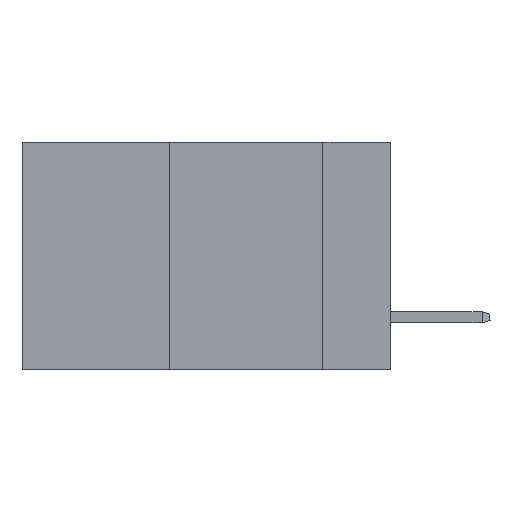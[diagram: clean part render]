
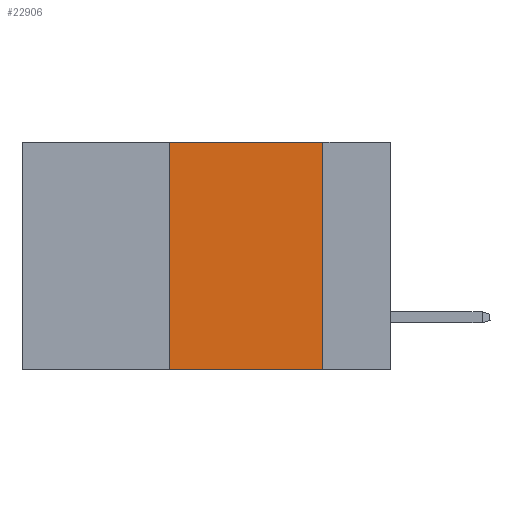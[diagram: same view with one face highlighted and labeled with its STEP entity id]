
A CAD part, left-side view. The second image highlights one B-rep face of the part: STEP entity #22906.
In plain terms, the highlighted planar face has unit normal (-1, 0, 0).
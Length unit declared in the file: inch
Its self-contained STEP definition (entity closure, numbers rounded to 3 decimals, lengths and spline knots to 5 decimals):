
#1070 = DIRECTION ( 'NONE',  ( 0., 0., 1. ) ) ;
#1856 = LINE ( 'NONE', #33654, #6864 ) ;
#2321 = CARTESIAN_POINT ( 'NONE',  ( 0., 0.6, -0.37 ) ) ;
#2967 = EDGE_CURVE ( 'NONE', #23604, #9490, #24756, .T. ) ;
#3745 = FACE_OUTER_BOUND ( 'NONE', #18576, .T. ) ;
#4186 = LINE ( 'NONE', #20845, #26300 ) ;
#4460 = DIRECTION ( 'NONE',  ( 1., 0., 0. ) ) ;
#4631 = EDGE_CURVE ( 'NONE', #9490, #32981, #4186, .T. ) ;
#6123 = EDGE_CURVE ( 'NONE', #23604, #20145, #26373, .T. ) ;
#6767 = DIRECTION ( 'NONE',  ( 0., 0., -1. ) ) ;
#6864 = VECTOR ( 'NONE', #6767, 39.37008 ) ;
#7736 = DIRECTION ( 'NONE',  ( 0., -1., 0. ) ) ;
#9490 = VERTEX_POINT ( 'NONE', #29292 ) ;
#10195 = VECTOR ( 'NONE', #7736, 39.37008 ) ;
#12508 = CARTESIAN_POINT ( 'NONE',  ( 0., 0.6, 0. ) ) ;
#13231 = ORIENTED_EDGE ( 'NONE', *, *, #25130, .F. ) ;
#15434 = ORIENTED_EDGE ( 'NONE', *, *, #4631, .F. ) ;
#16707 = CARTESIAN_POINT ( 'NONE',  ( 0., 0.11, 0. ) ) ;
#17453 = ORIENTED_EDGE ( 'NONE', *, *, #2967, .F. ) ;
#17587 = VECTOR ( 'NONE', #1070, 39.37008 ) ;
#18473 = CARTESIAN_POINT ( 'NONE',  ( 0., 0.11, -0.37 ) ) ;
#18576 = EDGE_LOOP ( 'NONE', ( #13231, #15434, #17453, #18637 ) ) ;
#18637 = ORIENTED_EDGE ( 'NONE', *, *, #6123, .T. ) ;
#20145 = VERTEX_POINT ( 'NONE', #18473 ) ;
#20845 = CARTESIAN_POINT ( 'NONE',  ( 0., 0.6, 0. ) ) ;
#22906 = ADVANCED_FACE ( 'NONE', ( #3745 ), #33245, .F. ) ;
#23501 = DIRECTION ( 'NONE',  ( 0., -1., 0. ) ) ;
#23604 = VERTEX_POINT ( 'NONE', #29286 ) ;
#24595 = CARTESIAN_POINT ( 'NONE',  ( 0., 0.36, 0. ) ) ;
#24756 = LINE ( 'NONE', #24595, #17587 ) ;
#25130 = EDGE_CURVE ( 'NONE', #32981, #20145, #1856, .T. ) ;
#26300 = VECTOR ( 'NONE', #23501, 39.37008 ) ;
#26373 = LINE ( 'NONE', #2321, #10195 ) ;
#28334 = DIRECTION ( 'NONE',  ( 0., 0., -1. ) ) ;
#29286 = CARTESIAN_POINT ( 'NONE',  ( 0., 0.36, -0.37 ) ) ;
#29292 = CARTESIAN_POINT ( 'NONE',  ( 0., 0.36, 0. ) ) ;
#31344 = AXIS2_PLACEMENT_3D ( 'NONE', #12508, #4460, #28334 ) ;
#32981 = VERTEX_POINT ( 'NONE', #16707 ) ;
#33245 = PLANE ( 'NONE',  #31344 ) ;
#33654 = CARTESIAN_POINT ( 'NONE',  ( 0., 0.11, 0. ) ) ;
